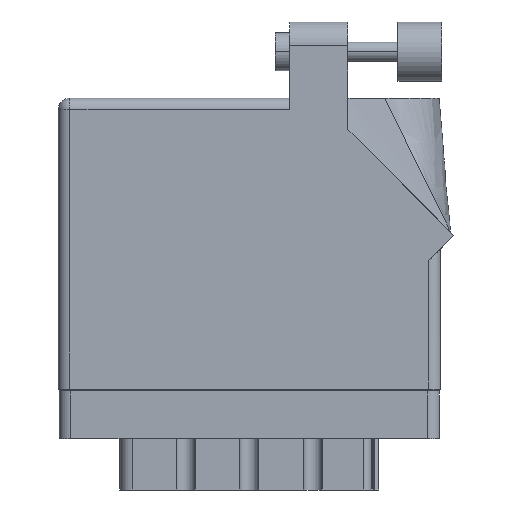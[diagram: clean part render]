
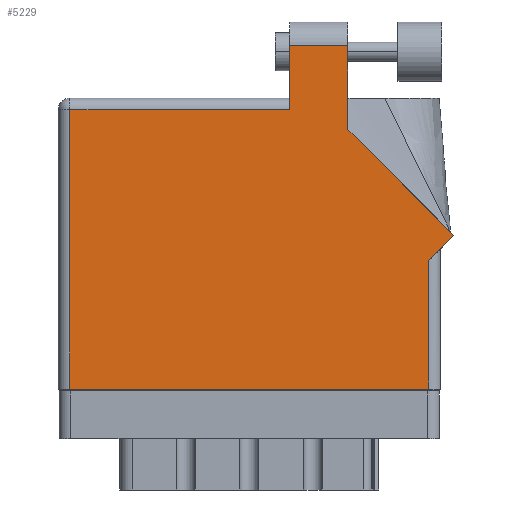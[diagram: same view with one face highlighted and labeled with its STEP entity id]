
A CAD part, front view. The second image highlights one B-rep face of the part: STEP entity #5229.
In plain terms, the highlighted face is planar.
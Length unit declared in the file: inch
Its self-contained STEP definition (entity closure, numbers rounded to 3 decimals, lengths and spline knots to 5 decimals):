
#1301 = ORIENTED_EDGE ( 'NONE', *, *, #30627, .T. ) ;
#1420 = CARTESIAN_POINT ( 'NONE',  ( 1.948, 0.737, 0. ) ) ;
#1521 = CARTESIAN_POINT ( 'NONE',  ( 0.062, 1.468, 0. ) ) ;
#3102 = LINE ( 'NONE', #34191, #31950 ) ;
#3610 = VECTOR ( 'NONE', #17859, 39.37008 ) ;
#3761 = VECTOR ( 'NONE', #40947, 39.37008 ) ;
#3957 = CARTESIAN_POINT ( 'NONE',  ( 1.217, 1.805, 0. ) ) ;
#4211 = LINE ( 'NONE', #1420, #5206 ) ;
#4421 = ORIENTED_EDGE ( 'NONE', *, *, #10995, .T. ) ;
#4872 = VECTOR ( 'NONE', #11704, 39.37008 ) ;
#5206 = VECTOR ( 'NONE', #29932, 39.37008 ) ;
#5229 = ADVANCED_FACE ( 'NONE', ( #27886 ), #22324, .F. ) ;
#5907 = AXIS2_PLACEMENT_3D ( 'NONE', #25652, #13156, #38067 ) ;
#9366 = ORIENTED_EDGE ( 'NONE', *, *, #28449, .T. ) ;
#9456 = VECTOR ( 'NONE', #19349, 39.37008 ) ;
#9736 = LINE ( 'NONE', #18519, #3761 ) ;
#10281 = EDGE_CURVE ( 'NONE', #30539, #40326, #33758, .T. ) ;
#10435 = ORIENTED_EDGE ( 'NONE', *, *, #21689, .T. ) ;
#10995 = EDGE_CURVE ( 'NONE', #31815, #17348, #11774, .T. ) ;
#11129 = EDGE_CURVE ( 'NONE', #21650, #20362, #12777, .T. ) ;
#11704 = DIRECTION ( 'NONE',  ( 0., -1., 0. ) ) ;
#11774 = LINE ( 'NONE', #3957, #26671 ) ;
#12064 = LINE ( 'NONE', #17580, #3610 ) ;
#12134 = EDGE_LOOP ( 'NONE', ( #33486, #4421, #1301, #9366, #37212, #15132, #12280, #27724, #10435 ) ) ;
#12280 = ORIENTED_EDGE ( 'NONE', *, *, #37494, .T. ) ;
#12777 = LINE ( 'NONE', #39983, #20191 ) ;
#13156 = DIRECTION ( 'NONE',  ( 0., 0., -1. ) ) ;
#14539 = VERTEX_POINT ( 'NONE', #26447 ) ;
#15132 = ORIENTED_EDGE ( 'NONE', *, *, #17150, .T. ) ;
#16727 = CARTESIAN_POINT ( 'NONE',  ( 2.08071, 0.80771, 0. ) ) ;
#17150 = EDGE_CURVE ( 'NONE', #40326, #14539, #30396, .T. ) ;
#17348 = VERTEX_POINT ( 'NONE', #24266 ) ;
#17580 = CARTESIAN_POINT ( 'NONE',  ( 2.08071, 0.80771, 0. ) ) ;
#17859 = DIRECTION ( 'NONE',  ( -0.707, 0.707, 0. ) ) ;
#18516 = CARTESIAN_POINT ( 'NONE',  ( 1.524, 1.805, 0. ) ) ;
#18519 = CARTESIAN_POINT ( 'NONE',  ( 1.217, 1.53, 0. ) ) ;
#19211 = CARTESIAN_POINT ( 'NONE',  ( 0., 1.468, 0. ) ) ;
#19349 = DIRECTION ( 'NONE',  ( -1., 0., 0. ) ) ;
#19564 = CARTESIAN_POINT ( 'NONE',  ( 1.217, 1.468, 0. ) ) ;
#20191 = VECTOR ( 'NONE', #36467, 39.37008 ) ;
#20362 = VERTEX_POINT ( 'NONE', #16727 ) ;
#21650 = VERTEX_POINT ( 'NONE', #39317 ) ;
#21689 = EDGE_CURVE ( 'NONE', #20362, #23273, #12064, .T. ) ;
#22324 = PLANE ( 'NONE',  #5907 ) ;
#23273 = VERTEX_POINT ( 'NONE', #38052 ) ;
#23879 = LINE ( 'NONE', #19211, #9456 ) ;
#24266 = CARTESIAN_POINT ( 'NONE',  ( 1.217, 1.805, 0. ) ) ;
#25652 = CARTESIAN_POINT ( 'NONE',  ( 0., 1.53, 0. ) ) ;
#26447 = CARTESIAN_POINT ( 'NONE',  ( 1.948, 0., 0. ) ) ;
#26671 = VECTOR ( 'NONE', #35760, 39.37008 ) ;
#27724 = ORIENTED_EDGE ( 'NONE', *, *, #11129, .T. ) ;
#27886 = FACE_OUTER_BOUND ( 'NONE', #12134, .T. ) ;
#28279 = CARTESIAN_POINT ( 'NONE',  ( 0.062, 0., 0. ) ) ;
#28449 = EDGE_CURVE ( 'NONE', #30765, #30539, #23879, .T. ) ;
#29901 = VECTOR ( 'NONE', #33050, 39.37008 ) ;
#29932 = DIRECTION ( 'NONE',  ( 0., 1., 0. ) ) ;
#30396 = LINE ( 'NONE', #33604, #29901 ) ;
#30539 = VERTEX_POINT ( 'NONE', #1521 ) ;
#30627 = EDGE_CURVE ( 'NONE', #17348, #30765, #9736, .T. ) ;
#30765 = VERTEX_POINT ( 'NONE', #19564 ) ;
#31815 = VERTEX_POINT ( 'NONE', #18516 ) ;
#31950 = VECTOR ( 'NONE', #33921, 39.37008 ) ;
#32303 = EDGE_CURVE ( 'NONE', #23273, #31815, #3102, .T. ) ;
#33050 = DIRECTION ( 'NONE',  ( 1., 0., 0. ) ) ;
#33486 = ORIENTED_EDGE ( 'NONE', *, *, #32303, .T. ) ;
#33604 = CARTESIAN_POINT ( 'NONE',  ( 0., 0., 0. ) ) ;
#33758 = LINE ( 'NONE', #39832, #4872 ) ;
#33921 = DIRECTION ( 'NONE',  ( 0., 1., 0. ) ) ;
#34191 = CARTESIAN_POINT ( 'NONE',  ( 1.524, 1.36442, 0. ) ) ;
#35760 = DIRECTION ( 'NONE',  ( -1., 0., 0. ) ) ;
#36467 = DIRECTION ( 'NONE',  ( 0.707, 0.707, 0. ) ) ;
#37212 = ORIENTED_EDGE ( 'NONE', *, *, #10281, .T. ) ;
#37494 = EDGE_CURVE ( 'NONE', #14539, #21650, #4211, .T. ) ;
#38052 = CARTESIAN_POINT ( 'NONE',  ( 1.524, 1.36442, 0. ) ) ;
#38067 = DIRECTION ( 'NONE',  ( -1., 0., 0. ) ) ;
#39317 = CARTESIAN_POINT ( 'NONE',  ( 1.948, 0.675, 0. ) ) ;
#39832 = CARTESIAN_POINT ( 'NONE',  ( 0.062, 0., 0. ) ) ;
#39983 = CARTESIAN_POINT ( 'NONE',  ( 2.01, 0.737, 0. ) ) ;
#40326 = VERTEX_POINT ( 'NONE', #28279 ) ;
#40947 = DIRECTION ( 'NONE',  ( 0., -1., 0. ) ) ;
